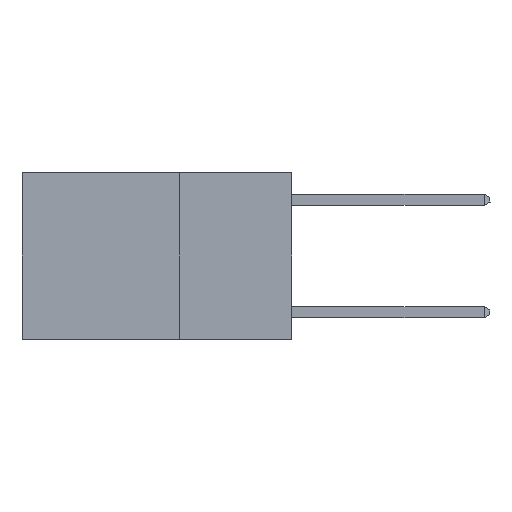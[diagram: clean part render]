
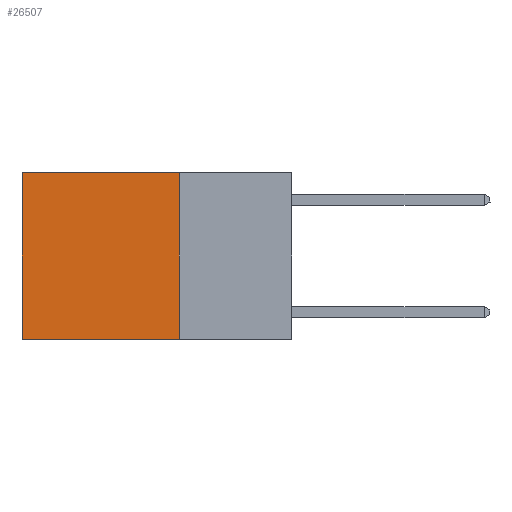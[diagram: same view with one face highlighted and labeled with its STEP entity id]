
A CAD part, left-side view. The second image highlights one B-rep face of the part: STEP entity #26507.
In plain terms, the highlighted planar face has unit normal (-1, 0, 0).
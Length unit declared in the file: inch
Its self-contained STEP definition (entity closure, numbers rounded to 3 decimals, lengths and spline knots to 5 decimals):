
#214 = VERTEX_POINT ( 'NONE', #5923 ) ;
#3635 = CARTESIAN_POINT ( 'NONE',  ( 0.2625, 0.6, 0. ) ) ;
#5923 = CARTESIAN_POINT ( 'NONE',  ( 0.2625, 0.25, -0.37 ) ) ;
#6753 = ORIENTED_EDGE ( 'NONE', *, *, #21925, .F. ) ;
#8119 = VERTEX_POINT ( 'NONE', #19610 ) ;
#8322 = CARTESIAN_POINT ( 'NONE',  ( 0.2625, 0.25, 0. ) ) ;
#8790 = CARTESIAN_POINT ( 'NONE',  ( 0.2625, 0.6, -0.37 ) ) ;
#9158 = EDGE_CURVE ( 'NONE', #8119, #18715, #29899, .T. ) ;
#9830 = EDGE_CURVE ( 'NONE', #214, #20467, #28551, .T. ) ;
#9852 = CARTESIAN_POINT ( 'NONE',  ( 0.2625, 0.25, -0.37 ) ) ;
#9905 = CARTESIAN_POINT ( 'NONE',  ( 0.2625, 0.6, 0. ) ) ;
#11173 = FACE_OUTER_BOUND ( 'NONE', #16783, .T. ) ;
#14220 = DIRECTION ( 'NONE',  ( 0., 1., 0. ) ) ;
#15831 = DIRECTION ( 'NONE',  ( 0., 0., -1. ) ) ;
#16207 = CARTESIAN_POINT ( 'NONE',  ( 0.2625, 0.25, 0. ) ) ;
#16783 = EDGE_LOOP ( 'NONE', ( #26688, #21770, #6753, #20873 ) ) ;
#18425 = VECTOR ( 'NONE', #15831, 39.37008 ) ;
#18715 = VERTEX_POINT ( 'NONE', #3635 ) ;
#19610 = CARTESIAN_POINT ( 'NONE',  ( 0.2625, 0.25, 0. ) ) ;
#20236 = LINE ( 'NONE', #29216, #18425 ) ;
#20467 = VERTEX_POINT ( 'NONE', #8790 ) ;
#20873 = ORIENTED_EDGE ( 'NONE', *, *, #9158, .T. ) ;
#21716 = DIRECTION ( 'NONE',  ( 1., 0., 0. ) ) ;
#21770 = ORIENTED_EDGE ( 'NONE', *, *, #9830, .F. ) ;
#21876 = DIRECTION ( 'NONE',  ( 0., 0., -1. ) ) ;
#21925 = EDGE_CURVE ( 'NONE', #8119, #214, #20236, .T. ) ;
#23444 = LINE ( 'NONE', #9905, #26316 ) ;
#25400 = VECTOR ( 'NONE', #14220, 39.37008 ) ;
#25476 = VECTOR ( 'NONE', #28111, 39.37008 ) ;
#26316 = VECTOR ( 'NONE', #28316, 39.37008 ) ;
#26507 = ADVANCED_FACE ( 'NONE', ( #11173 ), #29744, .F. ) ;
#26688 = ORIENTED_EDGE ( 'NONE', *, *, #27146, .T. ) ;
#27146 = EDGE_CURVE ( 'NONE', #18715, #20467, #23444, .T. ) ;
#28111 = DIRECTION ( 'NONE',  ( 0., 1., 0. ) ) ;
#28316 = DIRECTION ( 'NONE',  ( 0., 0., -1. ) ) ;
#28551 = LINE ( 'NONE', #9852, #25476 ) ;
#29205 = AXIS2_PLACEMENT_3D ( 'NONE', #8322, #21716, #21876 ) ;
#29216 = CARTESIAN_POINT ( 'NONE',  ( 0.2625, 0.25, 0. ) ) ;
#29744 = PLANE ( 'NONE',  #29205 ) ;
#29899 = LINE ( 'NONE', #16207, #25400 ) ;
